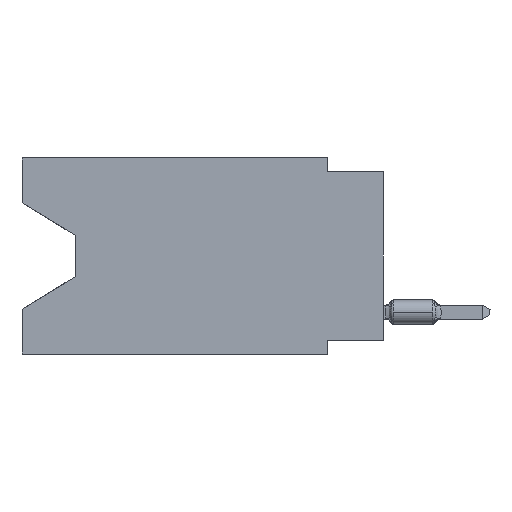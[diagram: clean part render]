
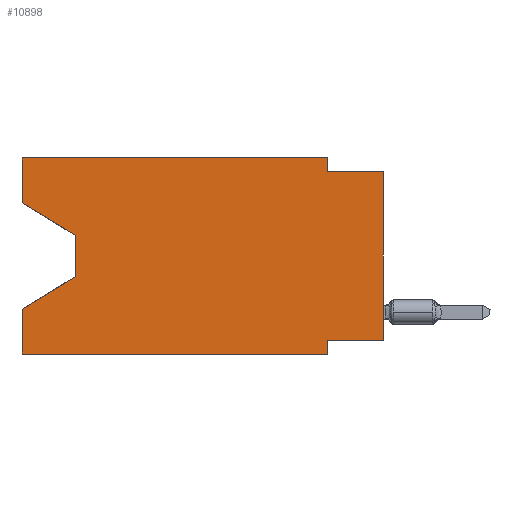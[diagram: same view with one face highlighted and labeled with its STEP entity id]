
A CAD part, left-side view. The second image highlights one B-rep face of the part: STEP entity #10898.
In plain terms, the highlighted planar face has unit normal (-1, 0, 0).
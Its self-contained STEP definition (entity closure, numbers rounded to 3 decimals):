
#6 = DIRECTION ( 'NONE',  ( 0., -1., 0. ) ) ;
#522 = EDGE_CURVE ( 'NONE', #19899, #18528, #1383, .T. ) ;
#530 = ORIENTED_EDGE ( 'NONE', *, *, #7119, .F. ) ;
#1383 = LINE ( 'NONE', #5181, #15155 ) ;
#1684 = CARTESIAN_POINT ( 'NONE',  ( 0., 16.383, -2.038 ) ) ;
#1817 = VECTOR ( 'NONE', #25134, 1000. ) ;
#2057 = VECTOR ( 'NONE', #6, 1000. ) ;
#2549 = VECTOR ( 'NONE', #21538, 1000. ) ;
#2561 = EDGE_CURVE ( 'NONE', #7274, #6303, #23421, .T. ) ;
#2666 = ORIENTED_EDGE ( 'NONE', *, *, #22693, .T. ) ;
#2933 = EDGE_CURVE ( 'NONE', #25222, #18297, #19446, .T. ) ;
#3013 = CARTESIAN_POINT ( 'NONE',  ( 0., 13.97, -3.505 ) ) ;
#3597 = ORIENTED_EDGE ( 'NONE', *, *, #21299, .F. ) ;
#4035 = VERTEX_POINT ( 'NONE', #13243 ) ;
#4383 = DIRECTION ( 'NONE',  ( 0., 0.855, -0.519 ) ) ;
#4763 = VECTOR ( 'NONE', #8570, 1000. ) ;
#5181 = CARTESIAN_POINT ( 'NONE',  ( 0., 16.383, 0. ) ) ;
#5451 = CARTESIAN_POINT ( 'NONE',  ( 0., 16.383, -8.89 ) ) ;
#5508 = DIRECTION ( 'NONE',  ( 0., 0., -1. ) ) ;
#5639 = DIRECTION ( 'NONE',  ( 0., 0., 1. ) ) ;
#5646 = LINE ( 'NONE', #9957, #2057 ) ;
#5688 = CARTESIAN_POINT ( 'NONE',  ( 0., 16.383, 0. ) ) ;
#5694 = ORIENTED_EDGE ( 'NONE', *, *, #15212, .F. ) ;
#6273 = ORIENTED_EDGE ( 'NONE', *, *, #2933, .T. ) ;
#6303 = VERTEX_POINT ( 'NONE', #6835 ) ;
#6835 = CARTESIAN_POINT ( 'NONE',  ( 0., 13.97, -5.385 ) ) ;
#7119 = EDGE_CURVE ( 'NONE', #18415, #21134, #23497, .T. ) ;
#7209 = ORIENTED_EDGE ( 'NONE', *, *, #522, .F. ) ;
#7274 = VERTEX_POINT ( 'NONE', #22819 ) ;
#7458 = CARTESIAN_POINT ( 'NONE',  ( 0., 2.54, -8.89 ) ) ;
#7728 = VECTOR ( 'NONE', #15128, 1000. ) ;
#7733 = VERTEX_POINT ( 'NONE', #24100 ) ;
#7972 = CARTESIAN_POINT ( 'NONE',  ( 0., 16.383, 0. ) ) ;
#8197 = VECTOR ( 'NONE', #5639, 1000. ) ;
#8570 = DIRECTION ( 'NONE',  ( 0., 0., -1. ) ) ;
#9364 = AXIS2_PLACEMENT_3D ( 'NONE', #24177, #20500, #22470 ) ;
#9957 = CARTESIAN_POINT ( 'NONE',  ( 0., 16.383, 0. ) ) ;
#10051 = DIRECTION ( 'NONE',  ( 0., 0., -1. ) ) ;
#10103 = VECTOR ( 'NONE', #21548, 1000. ) ;
#10274 = EDGE_CURVE ( 'NONE', #11524, #7733, #21365, .T. ) ;
#10389 = CARTESIAN_POINT ( 'NONE',  ( 0., 13.97, -5.385 ) ) ;
#10560 = PLANE ( 'NONE',  #9364 ) ;
#10662 = VECTOR ( 'NONE', #4383, 1000. ) ;
#10866 = VECTOR ( 'NONE', #5508, 1000. ) ;
#10898 = ADVANCED_FACE ( 'NONE', ( #24052 ), #10560, .F. ) ;
#11231 = CARTESIAN_POINT ( 'NONE',  ( 0., 2.54, -0.635 ) ) ;
#11373 = CARTESIAN_POINT ( 'NONE',  ( 0., 0., -8.255 ) ) ;
#11524 = VERTEX_POINT ( 'NONE', #11231 ) ;
#11571 = LINE ( 'NONE', #5688, #24576 ) ;
#11889 = CARTESIAN_POINT ( 'NONE',  ( 0., 2.54, 0. ) ) ;
#12009 = LINE ( 'NONE', #19991, #24595 ) ;
#12038 = LINE ( 'NONE', #19758, #8197 ) ;
#12130 = LINE ( 'NONE', #18264, #4763 ) ;
#12687 = VERTEX_POINT ( 'NONE', #11889 ) ;
#13155 = DIRECTION ( 'NONE',  ( 0., 0., 1. ) ) ;
#13243 = CARTESIAN_POINT ( 'NONE',  ( 0., 16.383, -6.852 ) ) ;
#14548 = ORIENTED_EDGE ( 'NONE', *, *, #19526, .T. ) ;
#15128 = DIRECTION ( 'NONE',  ( 0., -0.855, -0.519 ) ) ;
#15155 = VECTOR ( 'NONE', #13155, 1000. ) ;
#15212 = EDGE_CURVE ( 'NONE', #18528, #12687, #5646, .T. ) ;
#15527 = CARTESIAN_POINT ( 'NONE',  ( 0., 0., -8.255 ) ) ;
#15799 = EDGE_CURVE ( 'NONE', #21134, #18297, #12009, .T. ) ;
#16143 = ORIENTED_EDGE ( 'NONE', *, *, #15799, .F. ) ;
#16315 = EDGE_CURVE ( 'NONE', #25222, #4035, #11571, .T. ) ;
#17219 = CARTESIAN_POINT ( 'NONE',  ( 0., 16.383, -2.038 ) ) ;
#17260 = CARTESIAN_POINT ( 'NONE',  ( 0., 16.383, -8.89 ) ) ;
#17438 = CARTESIAN_POINT ( 'NONE',  ( 0., 0., -0.635 ) ) ;
#17584 = ORIENTED_EDGE ( 'NONE', *, *, #16315, .F. ) ;
#18264 = CARTESIAN_POINT ( 'NONE',  ( 0., 2.54, 0. ) ) ;
#18297 = VERTEX_POINT ( 'NONE', #7458 ) ;
#18415 = VERTEX_POINT ( 'NONE', #11373 ) ;
#18528 = VERTEX_POINT ( 'NONE', #7972 ) ;
#19177 = EDGE_LOOP ( 'NONE', ( #2666, #24898, #21952, #17584, #6273, #16143, #530, #14548, #24565, #3597, #5694, #7209 ) ) ;
#19446 = LINE ( 'NONE', #5451, #2549 ) ;
#19476 = CARTESIAN_POINT ( 'NONE',  ( 0., 2.54, -8.255 ) ) ;
#19526 = EDGE_CURVE ( 'NONE', #18415, #7733, #12038, .T. ) ;
#19758 = CARTESIAN_POINT ( 'NONE',  ( 0., 0., 0. ) ) ;
#19899 = VERTEX_POINT ( 'NONE', #1684 ) ;
#19991 = CARTESIAN_POINT ( 'NONE',  ( 0., 2.54, -8.89 ) ) ;
#20500 = DIRECTION ( 'NONE',  ( 1., 0., 0. ) ) ;
#20748 = LINE ( 'NONE', #17219, #7728 ) ;
#21134 = VERTEX_POINT ( 'NONE', #19476 ) ;
#21299 = EDGE_CURVE ( 'NONE', #12687, #11524, #12130, .T. ) ;
#21365 = LINE ( 'NONE', #17438, #1817 ) ;
#21386 = DIRECTION ( 'NONE',  ( 0., 0., 1. ) ) ;
#21538 = DIRECTION ( 'NONE',  ( 0., -1., 0. ) ) ;
#21548 = DIRECTION ( 'NONE',  ( 0., 1., 0. ) ) ;
#21952 = ORIENTED_EDGE ( 'NONE', *, *, #23030, .T. ) ;
#22470 = DIRECTION ( 'NONE',  ( 0., 0., -1. ) ) ;
#22693 = EDGE_CURVE ( 'NONE', #19899, #7274, #20748, .T. ) ;
#22819 = CARTESIAN_POINT ( 'NONE',  ( 0., 13.97, -3.505 ) ) ;
#23030 = EDGE_CURVE ( 'NONE', #6303, #4035, #24766, .T. ) ;
#23421 = LINE ( 'NONE', #3013, #10866 ) ;
#23497 = LINE ( 'NONE', #15527, #10103 ) ;
#24052 = FACE_OUTER_BOUND ( 'NONE', #19177, .T. ) ;
#24100 = CARTESIAN_POINT ( 'NONE',  ( 0., 0., -0.635 ) ) ;
#24177 = CARTESIAN_POINT ( 'NONE',  ( 0., 16.383, 0. ) ) ;
#24565 = ORIENTED_EDGE ( 'NONE', *, *, #10274, .F. ) ;
#24576 = VECTOR ( 'NONE', #21386, 1000. ) ;
#24595 = VECTOR ( 'NONE', #10051, 1000. ) ;
#24766 = LINE ( 'NONE', #10389, #10662 ) ;
#24898 = ORIENTED_EDGE ( 'NONE', *, *, #2561, .T. ) ;
#25134 = DIRECTION ( 'NONE',  ( 0., -1., 0. ) ) ;
#25222 = VERTEX_POINT ( 'NONE', #17260 ) ;
